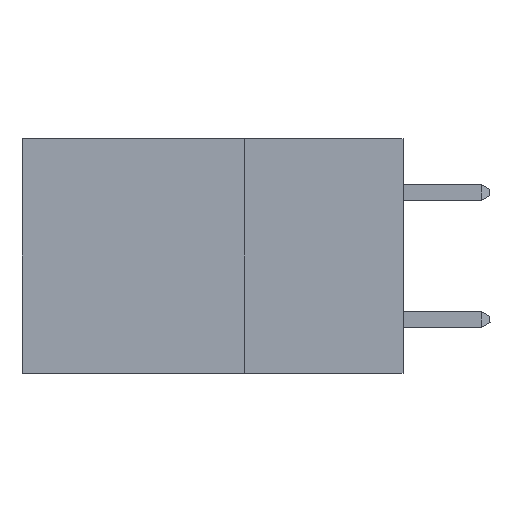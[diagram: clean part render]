
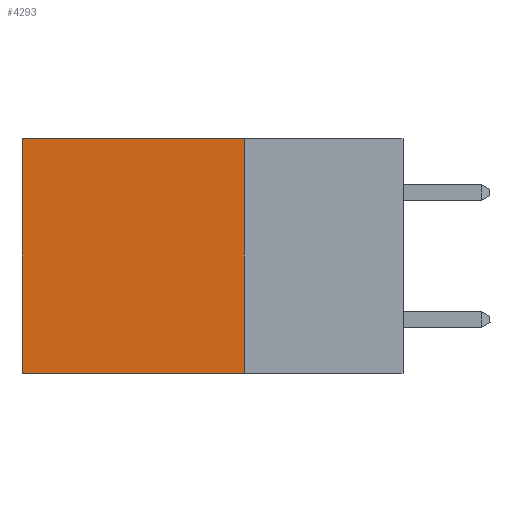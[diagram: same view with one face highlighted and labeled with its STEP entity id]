
A CAD part, left-side view. The second image highlights one B-rep face of the part: STEP entity #4293.
In plain terms, the highlighted planar face has unit normal (-1, 0, 0).
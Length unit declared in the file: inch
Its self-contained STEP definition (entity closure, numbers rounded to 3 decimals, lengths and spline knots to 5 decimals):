
#344 = VERTEX_POINT ( 'NONE', #12765 ) ;
#640 = EDGE_CURVE ( 'NONE', #12978, #344, #12313, .T. ) ;
#796 = AXIS2_PLACEMENT_3D ( 'NONE', #13562, #4820, #5011 ) ;
#1623 = ORIENTED_EDGE ( 'NONE', *, *, #8680, .F. ) ;
#1651 = DIRECTION ( 'NONE',  ( 0., 1., 0. ) ) ;
#1697 = PLANE ( 'NONE',  #796 ) ;
#1748 = EDGE_CURVE ( 'NONE', #6668, #12978, #5018, .T. ) ;
#2116 = LINE ( 'NONE', #7449, #2455 ) ;
#2129 = VECTOR ( 'NONE', #13905, 39.37008 ) ;
#2455 = VECTOR ( 'NONE', #9702, 39.37008 ) ;
#2740 = EDGE_LOOP ( 'NONE', ( #8228, #1623, #3352, #3190 ) ) ;
#3053 = FACE_OUTER_BOUND ( 'NONE', #2740, .T. ) ;
#3190 = ORIENTED_EDGE ( 'NONE', *, *, #1748, .T. ) ;
#3352 = ORIENTED_EDGE ( 'NONE', *, *, #9331, .F. ) ;
#4293 = ADVANCED_FACE ( 'NONE', ( #3053 ), #1697, .F. ) ;
#4505 = LINE ( 'NONE', #4729, #9928 ) ;
#4729 = CARTESIAN_POINT ( 'NONE',  ( 0.2875, 0.25, -0.37 ) ) ;
#4820 = DIRECTION ( 'NONE',  ( 1., 0., 0. ) ) ;
#5011 = DIRECTION ( 'NONE',  ( 0., 0., -1. ) ) ;
#5018 = LINE ( 'NONE', #6276, #2129 ) ;
#6276 = CARTESIAN_POINT ( 'NONE',  ( 0.2875, 0.25, 0. ) ) ;
#6374 = CARTESIAN_POINT ( 'NONE',  ( 0.2875, 0.6, 0. ) ) ;
#6570 = VERTEX_POINT ( 'NONE', #11721 ) ;
#6668 = VERTEX_POINT ( 'NONE', #8330 ) ;
#6902 = VECTOR ( 'NONE', #8588, 39.37008 ) ;
#7449 = CARTESIAN_POINT ( 'NONE',  ( 0.2875, 0.25, 0. ) ) ;
#8228 = ORIENTED_EDGE ( 'NONE', *, *, #640, .T. ) ;
#8330 = CARTESIAN_POINT ( 'NONE',  ( 0.2875, 0.25, 0. ) ) ;
#8588 = DIRECTION ( 'NONE',  ( 0., 0., -1. ) ) ;
#8680 = EDGE_CURVE ( 'NONE', #6570, #344, #4505, .T. ) ;
#9331 = EDGE_CURVE ( 'NONE', #6668, #6570, #2116, .T. ) ;
#9702 = DIRECTION ( 'NONE',  ( 0., 0., -1. ) ) ;
#9928 = VECTOR ( 'NONE', #1651, 39.37008 ) ;
#11721 = CARTESIAN_POINT ( 'NONE',  ( 0.2875, 0.25, -0.37 ) ) ;
#12198 = CARTESIAN_POINT ( 'NONE',  ( 0.2875, 0.6, 0. ) ) ;
#12313 = LINE ( 'NONE', #6374, #6902 ) ;
#12765 = CARTESIAN_POINT ( 'NONE',  ( 0.2875, 0.6, -0.37 ) ) ;
#12978 = VERTEX_POINT ( 'NONE', #12198 ) ;
#13562 = CARTESIAN_POINT ( 'NONE',  ( 0.2875, 0.25, 0. ) ) ;
#13905 = DIRECTION ( 'NONE',  ( 0., 1., 0. ) ) ;
